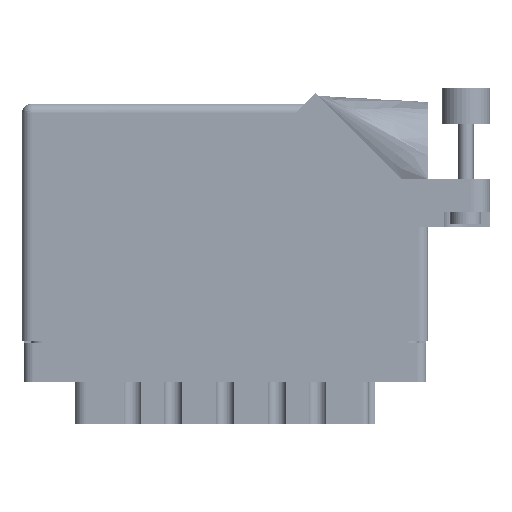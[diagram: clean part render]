
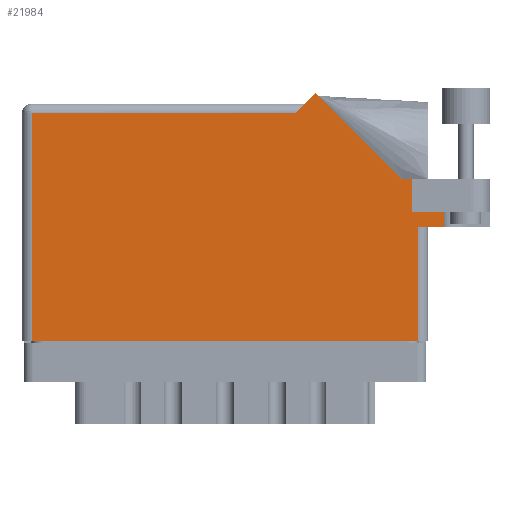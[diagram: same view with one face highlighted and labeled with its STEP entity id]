
A CAD part, front view. The second image highlights one B-rep face of the part: STEP entity #21984.
In plain terms, the highlighted face is planar.
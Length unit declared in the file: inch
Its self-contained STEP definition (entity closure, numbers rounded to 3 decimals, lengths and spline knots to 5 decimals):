
#304 = DIRECTION ( 'NONE',  ( -0.707, -0.707, 0. ) ) ;
#388 = CARTESIAN_POINT ( 'NONE',  ( 0.062, 0., 0. ) ) ;
#882 = CARTESIAN_POINT ( 'NONE',  ( 0., 0., 0. ) ) ;
#1306 = VERTEX_POINT ( 'NONE', #3453 ) ;
#3453 = CARTESIAN_POINT ( 'NONE',  ( 2.512, 1.044, 0. ) ) ;
#4088 = DIRECTION ( 'NONE',  ( 0., -1., 0. ) ) ;
#4603 = CARTESIAN_POINT ( 'NONE',  ( 2.512, 0.831, 0. ) ) ;
#4831 = ORIENTED_EDGE ( 'NONE', *, *, #10836, .T. ) ;
#5067 = ORIENTED_EDGE ( 'NONE', *, *, #23798, .T. ) ;
#6328 = LINE ( 'NONE', #39915, #22630 ) ;
#6363 = VERTEX_POINT ( 'NONE', #4603 ) ;
#6374 = ORIENTED_EDGE ( 'NONE', *, *, #47551, .T. ) ;
#7346 = EDGE_CURVE ( 'NONE', #10545, #42112, #37955, .T. ) ;
#7625 = DIRECTION ( 'NONE',  ( -1., 0., 0. ) ) ;
#8080 = CARTESIAN_POINT ( 'NONE',  ( 2.44642, 1.044, 0. ) ) ;
#8148 = CARTESIAN_POINT ( 'NONE',  ( 0., 1.468, 0. ) ) ;
#8840 = ORIENTED_EDGE ( 'NONE', *, *, #42342, .T. ) ;
#10194 = LINE ( 'NONE', #18946, #40242 ) ;
#10316 = VECTOR ( 'NONE', #4088, 39.37008 ) ;
#10486 = ORIENTED_EDGE ( 'NONE', *, *, #7346, .T. ) ;
#10545 = VERTEX_POINT ( 'NONE', #388 ) ;
#10836 = EDGE_CURVE ( 'NONE', #33389, #12203, #28831, .T. ) ;
#11268 = LINE ( 'NONE', #8080, #25029 ) ;
#12203 = VERTEX_POINT ( 'NONE', #53291 ) ;
#12260 = DIRECTION ( 'NONE',  ( -0.707, 0.707, 0. ) ) ;
#13435 = VECTOR ( 'NONE', #304, 39.37008 ) ;
#14470 = VECTOR ( 'NONE', #38964, 39.37008 ) ;
#15962 = CARTESIAN_POINT ( 'NONE',  ( 2.7135, 1.16177, 0. ) ) ;
#16332 = DIRECTION ( 'NONE',  ( 0., 1., 0. ) ) ;
#16340 = EDGE_LOOP ( 'NONE', ( #10486, #5067, #6374, #37936, #33684, #28324, #8840, #28237, #21846, #4831, #50660 ) ) ;
#16684 = CARTESIAN_POINT ( 'NONE',  ( 2.55, 0.737, 0. ) ) ;
#18148 = VERTEX_POINT ( 'NONE', #32670 ) ;
#18946 = CARTESIAN_POINT ( 'NONE',  ( 0.062, 0., 0. ) ) ;
#19079 = EDGE_CURVE ( 'NONE', #29142, #24484, #11268, .T. ) ;
#20371 = AXIS2_PLACEMENT_3D ( 'NONE', #24590, #33121, #7625 ) ;
#20392 = PLANE ( 'NONE',  #20371 ) ;
#21846 = ORIENTED_EDGE ( 'NONE', *, *, #29267, .T. ) ;
#21984 = ADVANCED_FACE ( 'NONE', ( #31273 ), #20392, .F. ) ;
#22143 = LINE ( 'NONE', #44867, #27414 ) ;
#22505 = EDGE_CURVE ( 'NONE', #18148, #24709, #42969, .T. ) ;
#22630 = VECTOR ( 'NONE', #48140, 39.37008 ) ;
#23798 = EDGE_CURVE ( 'NONE', #42112, #48357, #23918, .T. ) ;
#23918 = LINE ( 'NONE', #16684, #44834 ) ;
#24374 = EDGE_CURVE ( 'NONE', #12203, #10545, #10194, .T. ) ;
#24484 = VERTEX_POINT ( 'NONE', #34953 ) ;
#24565 = LINE ( 'NONE', #50489, #13435 ) ;
#24590 = CARTESIAN_POINT ( 'NONE',  ( 0., 1.53, 0. ) ) ;
#24709 = VERTEX_POINT ( 'NONE', #41553 ) ;
#25029 = VECTOR ( 'NONE', #12260, 39.37008 ) ;
#26229 = VECTOR ( 'NONE', #37667, 39.37008 ) ;
#26644 = CARTESIAN_POINT ( 'NONE',  ( 2.55, 0., 0. ) ) ;
#27010 = DIRECTION ( 'NONE',  ( 0., -1., 0. ) ) ;
#27033 = CARTESIAN_POINT ( 'NONE',  ( 1.757, 1.468, 0. ) ) ;
#27414 = VECTOR ( 'NONE', #36032, 39.37008 ) ;
#28237 = ORIENTED_EDGE ( 'NONE', *, *, #19079, .T. ) ;
#28324 = ORIENTED_EDGE ( 'NONE', *, *, #49563, .T. ) ;
#28735 = CARTESIAN_POINT ( 'NONE',  ( 2.55, 0.737, 0. ) ) ;
#28831 = LINE ( 'NONE', #8148, #26229 ) ;
#29142 = VERTEX_POINT ( 'NONE', #53053 ) ;
#29267 = EDGE_CURVE ( 'NONE', #24484, #33389, #24565, .T. ) ;
#31273 = FACE_OUTER_BOUND ( 'NONE', #16340, .T. ) ;
#32670 = CARTESIAN_POINT ( 'NONE',  ( 2.7135, 0.831, 0. ) ) ;
#33121 = DIRECTION ( 'NONE',  ( 0., 0., -1. ) ) ;
#33389 = VERTEX_POINT ( 'NONE', #27033 ) ;
#33684 = ORIENTED_EDGE ( 'NONE', *, *, #35872, .F. ) ;
#34953 = CARTESIAN_POINT ( 'NONE',  ( 1.88971, 1.60071, 0. ) ) ;
#35500 = LINE ( 'NONE', #39154, #44057 ) ;
#35872 = EDGE_CURVE ( 'NONE', #6363, #18148, #35500, .T. ) ;
#36032 = DIRECTION ( 'NONE',  ( 1., 0., 0. ) ) ;
#37667 = DIRECTION ( 'NONE',  ( -1., 0., 0. ) ) ;
#37936 = ORIENTED_EDGE ( 'NONE', *, *, #22505, .F. ) ;
#37955 = LINE ( 'NONE', #882, #14470 ) ;
#38964 = DIRECTION ( 'NONE',  ( 1., 0., 0. ) ) ;
#39154 = CARTESIAN_POINT ( 'NONE',  ( 2.512, 0.831, 0. ) ) ;
#39915 = CARTESIAN_POINT ( 'NONE',  ( 2.512, 0.831, 0. ) ) ;
#40242 = VECTOR ( 'NONE', #27010, 39.37008 ) ;
#41553 = CARTESIAN_POINT ( 'NONE',  ( 2.7135, 0.737, 0. ) ) ;
#42112 = VERTEX_POINT ( 'NONE', #26644 ) ;
#42342 = EDGE_CURVE ( 'NONE', #1306, #29142, #54118, .T. ) ;
#42969 = LINE ( 'NONE', #15962, #10316 ) ;
#42984 = VECTOR ( 'NONE', #53264, 39.37008 ) ;
#43377 = DIRECTION ( 'NONE',  ( 1., 0., 0. ) ) ;
#44057 = VECTOR ( 'NONE', #43377, 39.37008 ) ;
#44834 = VECTOR ( 'NONE', #16332, 39.37008 ) ;
#44867 = CARTESIAN_POINT ( 'NONE',  ( 2.612, 0.737, 0. ) ) ;
#47551 = EDGE_CURVE ( 'NONE', #48357, #24709, #22143, .T. ) ;
#48140 = DIRECTION ( 'NONE',  ( 0., 1., 0. ) ) ;
#48357 = VERTEX_POINT ( 'NONE', #28735 ) ;
#48850 = CARTESIAN_POINT ( 'NONE',  ( 3.012, 1.044, 0. ) ) ;
#49563 = EDGE_CURVE ( 'NONE', #6363, #1306, #6328, .T. ) ;
#50489 = CARTESIAN_POINT ( 'NONE',  ( 1.819, 1.53, 0. ) ) ;
#50660 = ORIENTED_EDGE ( 'NONE', *, *, #24374, .T. ) ;
#53053 = CARTESIAN_POINT ( 'NONE',  ( 2.44642, 1.044, 0. ) ) ;
#53264 = DIRECTION ( 'NONE',  ( -1., 0., 0. ) ) ;
#53291 = CARTESIAN_POINT ( 'NONE',  ( 0.062, 1.468, 0. ) ) ;
#54118 = LINE ( 'NONE', #48850, #42984 ) ;
